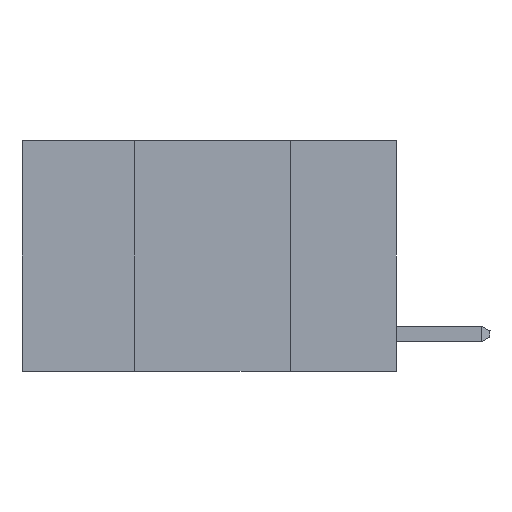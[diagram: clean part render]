
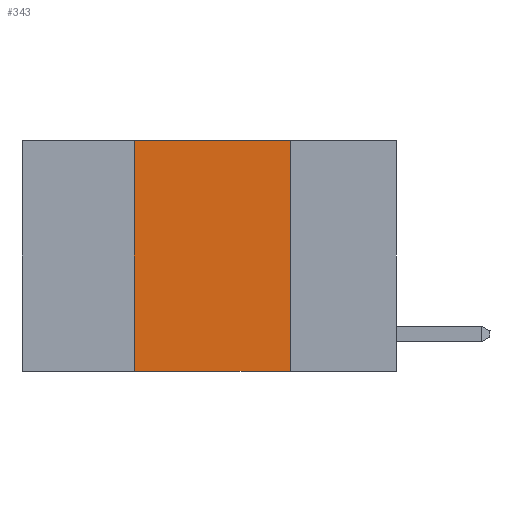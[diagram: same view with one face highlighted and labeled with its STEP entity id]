
A CAD part, left-side view. The second image highlights one B-rep face of the part: STEP entity #343.
In plain terms, the highlighted planar face has unit normal (-1, 0, 0).
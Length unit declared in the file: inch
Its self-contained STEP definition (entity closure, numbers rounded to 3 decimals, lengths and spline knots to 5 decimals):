
#58 = EDGE_CURVE ( 'NONE', #9377, #8635, #7555, .T. ) ;
#235 = EDGE_CURVE ( 'NONE', #8635, #3257, #3073, .T. ) ;
#343 = ADVANCED_FACE ( 'NONE', ( #4283 ), #10853, .F. ) ;
#2055 = CARTESIAN_POINT ( 'NONE',  ( 0., 0.17, 0. ) ) ;
#2253 = DIRECTION ( 'NONE',  ( 0., -1., 0. ) ) ;
#3073 = LINE ( 'NONE', #12445, #8014 ) ;
#3257 = VERTEX_POINT ( 'NONE', #5263 ) ;
#3382 = ORIENTED_EDGE ( 'NONE', *, *, #12588, .F. ) ;
#3427 = ORIENTED_EDGE ( 'NONE', *, *, #11634, .T. ) ;
#4283 = FACE_OUTER_BOUND ( 'NONE', #5300, .T. ) ;
#4376 = DIRECTION ( 'NONE',  ( 0., 0., -1. ) ) ;
#4390 = VECTOR ( 'NONE', #6545, 39.37008 ) ;
#4429 = CARTESIAN_POINT ( 'NONE',  ( 0., 0.6, -0.37 ) ) ;
#4929 = CARTESIAN_POINT ( 'NONE',  ( 0., 0.42, 0. ) ) ;
#5241 = VERTEX_POINT ( 'NONE', #6676 ) ;
#5263 = CARTESIAN_POINT ( 'NONE',  ( 0., 0.17, 0. ) ) ;
#5296 = DIRECTION ( 'NONE',  ( 0., 0., -1. ) ) ;
#5300 = EDGE_LOOP ( 'NONE', ( #3382, #8027, #9418, #3427 ) ) ;
#6545 = DIRECTION ( 'NONE',  ( 0., -1., 0. ) ) ;
#6648 = LINE ( 'NONE', #2055, #8697 ) ;
#6652 = CARTESIAN_POINT ( 'NONE',  ( 0., 0.6, 0. ) ) ;
#6676 = CARTESIAN_POINT ( 'NONE',  ( 0., 0.17, -0.37 ) ) ;
#6874 = AXIS2_PLACEMENT_3D ( 'NONE', #6652, #12641, #4376 ) ;
#7160 = LINE ( 'NONE', #4429, #4390 ) ;
#7555 = LINE ( 'NONE', #4929, #12402 ) ;
#7578 = DIRECTION ( 'NONE',  ( 0., 0., 1. ) ) ;
#8014 = VECTOR ( 'NONE', #2253, 39.37008 ) ;
#8027 = ORIENTED_EDGE ( 'NONE', *, *, #235, .F. ) ;
#8635 = VERTEX_POINT ( 'NONE', #9452 ) ;
#8697 = VECTOR ( 'NONE', #5296, 39.37008 ) ;
#9377 = VERTEX_POINT ( 'NONE', #9614 ) ;
#9418 = ORIENTED_EDGE ( 'NONE', *, *, #58, .F. ) ;
#9452 = CARTESIAN_POINT ( 'NONE',  ( 0., 0.42, 0. ) ) ;
#9614 = CARTESIAN_POINT ( 'NONE',  ( 0., 0.42, -0.37 ) ) ;
#10853 = PLANE ( 'NONE',  #6874 ) ;
#11634 = EDGE_CURVE ( 'NONE', #9377, #5241, #7160, .T. ) ;
#12402 = VECTOR ( 'NONE', #7578, 39.37008 ) ;
#12445 = CARTESIAN_POINT ( 'NONE',  ( 0., 0.6, 0. ) ) ;
#12588 = EDGE_CURVE ( 'NONE', #3257, #5241, #6648, .T. ) ;
#12641 = DIRECTION ( 'NONE',  ( 1., 0., 0. ) ) ;
